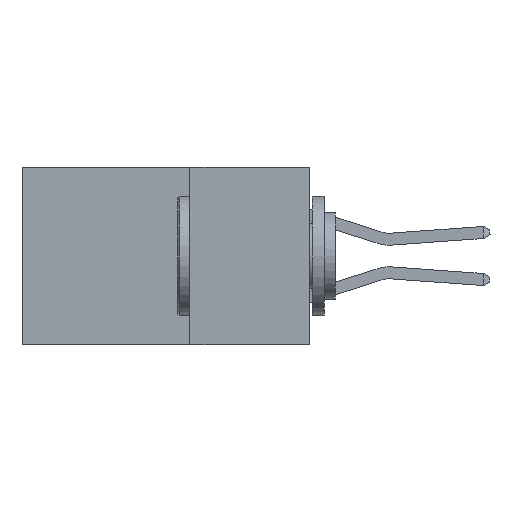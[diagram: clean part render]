
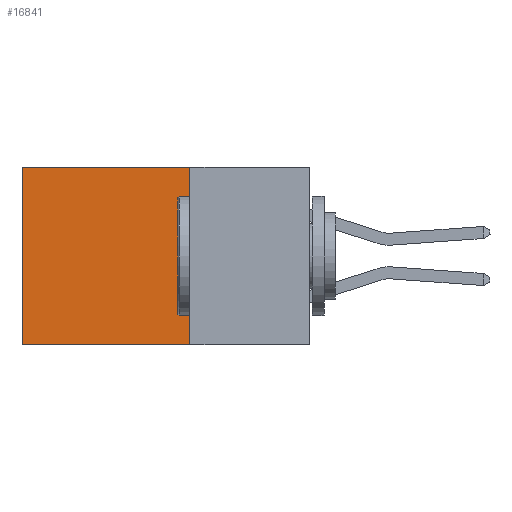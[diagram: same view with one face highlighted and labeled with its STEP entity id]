
A CAD part, left-side view. The second image highlights one B-rep face of the part: STEP entity #16841.
In plain terms, the highlighted planar face has unit normal (-1, 0, 0).
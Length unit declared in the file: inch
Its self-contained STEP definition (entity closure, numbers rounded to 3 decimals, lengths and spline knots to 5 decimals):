
#1034 = CARTESIAN_POINT ( 'NONE',  ( 0.2615, 0.25, 0. ) ) ;
#1515 = CARTESIAN_POINT ( 'NONE',  ( 0.2615, 0.6, -0.37 ) ) ;
#1940 = EDGE_LOOP ( 'NONE', ( #14343, #14206, #19087, #9515 ) ) ;
#2268 = VERTEX_POINT ( 'NONE', #1515 ) ;
#3101 = CARTESIAN_POINT ( 'NONE',  ( 0.2615, 0.25, -0.37 ) ) ;
#3149 = DIRECTION ( 'NONE',  ( 0., 0., -1. ) ) ;
#4094 = CARTESIAN_POINT ( 'NONE',  ( 0.2615, 0.25, 0. ) ) ;
#4800 = VERTEX_POINT ( 'NONE', #14636 ) ;
#4804 = VERTEX_POINT ( 'NONE', #4094 ) ;
#6544 = VECTOR ( 'NONE', #15011, 39.37008 ) ;
#7177 = EDGE_CURVE ( 'NONE', #4804, #22058, #16948, .T. ) ;
#7838 = CARTESIAN_POINT ( 'NONE',  ( 0.2615, 0.25, -0.37 ) ) ;
#8485 = DIRECTION ( 'NONE',  ( 0., 1., 0. ) ) ;
#9289 = EDGE_CURVE ( 'NONE', #4800, #2268, #9962, .T. ) ;
#9515 = ORIENTED_EDGE ( 'NONE', *, *, #17769, .T. ) ;
#9962 = LINE ( 'NONE', #11685, #6544 ) ;
#11685 = CARTESIAN_POINT ( 'NONE',  ( 0.2615, 0.6, -0.37 ) ) ;
#13029 = PLANE ( 'NONE',  #19677 ) ;
#13538 = LINE ( 'NONE', #1034, #17066 ) ;
#14206 = ORIENTED_EDGE ( 'NONE', *, *, #17260, .F. ) ;
#14343 = ORIENTED_EDGE ( 'NONE', *, *, #9289, .T. ) ;
#14636 = CARTESIAN_POINT ( 'NONE',  ( 0.2615, 0.6, 0. ) ) ;
#15011 = DIRECTION ( 'NONE',  ( 0., 0., -1. ) ) ;
#15221 = VECTOR ( 'NONE', #20861, 39.37008 ) ;
#16461 = FACE_OUTER_BOUND ( 'NONE', #1940, .T. ) ;
#16646 = DIRECTION ( 'NONE',  ( 0., 1., 0. ) ) ;
#16747 = VECTOR ( 'NONE', #16646, 39.37008 ) ;
#16841 = ADVANCED_FACE ( 'NONE', ( #16461 ), #13029, .F. ) ;
#16948 = LINE ( 'NONE', #18675, #15221 ) ;
#17066 = VECTOR ( 'NONE', #8485, 39.37008 ) ;
#17260 = EDGE_CURVE ( 'NONE', #22058, #2268, #21716, .T. ) ;
#17769 = EDGE_CURVE ( 'NONE', #4804, #4800, #13538, .T. ) ;
#18675 = CARTESIAN_POINT ( 'NONE',  ( 0.2615, 0.25, -0.37 ) ) ;
#19087 = ORIENTED_EDGE ( 'NONE', *, *, #7177, .F. ) ;
#19677 = AXIS2_PLACEMENT_3D ( 'NONE', #20024, #22529, #3149 ) ;
#20024 = CARTESIAN_POINT ( 'NONE',  ( 0.2615, 0.25, -0.37 ) ) ;
#20861 = DIRECTION ( 'NONE',  ( 0., 0., -1. ) ) ;
#21716 = LINE ( 'NONE', #7838, #16747 ) ;
#22058 = VERTEX_POINT ( 'NONE', #3101 ) ;
#22529 = DIRECTION ( 'NONE',  ( 1., 0., 0. ) ) ;
